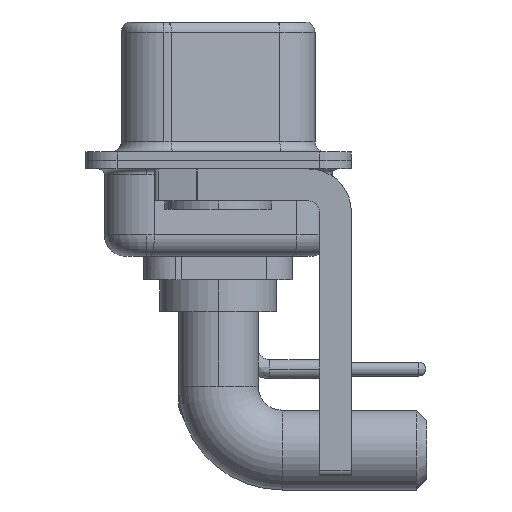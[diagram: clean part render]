
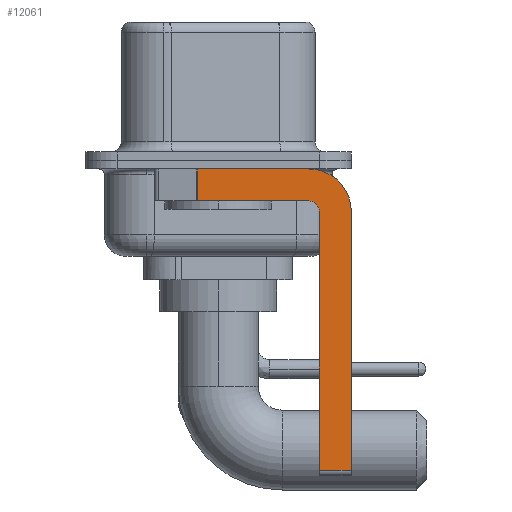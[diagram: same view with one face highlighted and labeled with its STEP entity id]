
A CAD part, left-side view. The second image highlights one B-rep face of the part: STEP entity #12061.
In plain terms, the highlighted planar face has unit normal (-1, 0, 0).
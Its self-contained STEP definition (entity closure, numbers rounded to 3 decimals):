
#58 = VERTEX_POINT ( 'NONE', #26443 ) ;
#80 = LINE ( 'NONE', #25278, #1724 ) ;
#83 = DIRECTION ( 'NONE',  ( 0., 0., -1. ) ) ;
#329 = VECTOR ( 'NONE', #21263, 1000. ) ;
#444 = CARTESIAN_POINT ( 'NONE',  ( -2.9, -4.25, -1.9 ) ) ;
#538 = CARTESIAN_POINT ( 'NONE',  ( -2.9, -4.75, -2.4 ) ) ;
#853 = DIRECTION ( 'NONE',  ( 0., 0., -1. ) ) ;
#1160 = ORIENTED_EDGE ( 'NONE', *, *, #6592, .F. ) ;
#1216 = DIRECTION ( 'NONE',  ( 0., 0., -1. ) ) ;
#1282 = CARTESIAN_POINT ( 'NONE',  ( -2.9, -6.25, -2.4 ) ) ;
#1724 = VECTOR ( 'NONE', #29143, 1000. ) ;
#2203 = EDGE_CURVE ( 'NONE', #13052, #23351, #20857, .T. ) ;
#2264 = EDGE_CURVE ( 'NONE', #17189, #18093, #7970, .T. ) ;
#3204 = CARTESIAN_POINT ( 'NONE',  ( -2.9, -4.25, -1.9 ) ) ;
#3882 = PLANE ( 'NONE',  #27304 ) ;
#5233 = VECTOR ( 'NONE', #12384, 1000. ) ;
#5284 = VERTEX_POINT ( 'NONE', #444 ) ;
#5597 = VERTEX_POINT ( 'NONE', #22332 ) ;
#5602 = CARTESIAN_POINT ( 'NONE',  ( -2.9, 0.978, -1.9 ) ) ;
#5744 = CARTESIAN_POINT ( 'NONE',  ( -2.9, -4.75, -14.8 ) ) ;
#6418 = ORIENTED_EDGE ( 'NONE', *, *, #2264, .F. ) ;
#6592 = EDGE_CURVE ( 'NONE', #5284, #23351, #21405, .T. ) ;
#7970 = LINE ( 'NONE', #5744, #10066 ) ;
#8335 = FACE_OUTER_BOUND ( 'NONE', #23864, .T. ) ;
#8390 = LINE ( 'NONE', #1282, #5233 ) ;
#8641 = EDGE_CURVE ( 'NONE', #58, #23050, #8390, .T. ) ;
#9135 = CARTESIAN_POINT ( 'NONE',  ( -2.9, -4.25, -2.4 ) ) ;
#9837 = ORIENTED_EDGE ( 'NONE', *, *, #27837, .F. ) ;
#10066 = VECTOR ( 'NONE', #14750, 1000. ) ;
#10176 = AXIS2_PLACEMENT_3D ( 'NONE', #28525, #28380, #28242 ) ;
#11211 = DIRECTION ( 'NONE',  ( 1., 0., 0. ) ) ;
#11667 = ORIENTED_EDGE ( 'NONE', *, *, #2203, .T. ) ;
#12061 = ADVANCED_FACE ( 'NONE', ( #8335 ), #3882, .F. ) ;
#12384 = DIRECTION ( 'NONE',  ( 0., 0., -1. ) ) ;
#13052 = VERTEX_POINT ( 'NONE', #17285 ) ;
#13055 = CARTESIAN_POINT ( 'NONE',  ( -2.9, -4.25, -2.4 ) ) ;
#14750 = DIRECTION ( 'NONE',  ( 0., 0., 1. ) ) ;
#15418 = LINE ( 'NONE', #21806, #25431 ) ;
#15426 = CIRCLE ( 'NONE', #18769, 2. ) ;
#17189 = VERTEX_POINT ( 'NONE', #27289 ) ;
#17285 = CARTESIAN_POINT ( 'NONE',  ( -2.9, 0.978, -0.4 ) ) ;
#17365 = DIRECTION ( 'NONE',  ( 1., 0., 0. ) ) ;
#17919 = EDGE_CURVE ( 'NONE', #13052, #5597, #15418, .T. ) ;
#18093 = VERTEX_POINT ( 'NONE', #538 ) ;
#18210 = CIRCLE ( 'NONE', #10176, 0.5 ) ;
#18769 = AXIS2_PLACEMENT_3D ( 'NONE', #9135, #11211, #83 ) ;
#19111 = CARTESIAN_POINT ( 'NONE',  ( -2.9, -6.25, -14.55 ) ) ;
#20632 = EDGE_CURVE ( 'NONE', #18093, #5284, #18210, .T. ) ;
#20857 = LINE ( 'NONE', #5602, #26624 ) ;
#21263 = DIRECTION ( 'NONE',  ( 0., 1., 0. ) ) ;
#21405 = LINE ( 'NONE', #3204, #329 ) ;
#21806 = CARTESIAN_POINT ( 'NONE',  ( -2.9, 3., -0.4 ) ) ;
#22332 = CARTESIAN_POINT ( 'NONE',  ( -2.9, -4.25, -0.4 ) ) ;
#23050 = VERTEX_POINT ( 'NONE', #19111 ) ;
#23351 = VERTEX_POINT ( 'NONE', #24565 ) ;
#23864 = EDGE_LOOP ( 'NONE', ( #26809, #11667, #1160, #28335, #6418, #25082, #28978, #9837 ) ) ;
#24304 = DIRECTION ( 'NONE',  ( 0., -1., 0. ) ) ;
#24565 = CARTESIAN_POINT ( 'NONE',  ( -2.9, 0.978, -1.9 ) ) ;
#25082 = ORIENTED_EDGE ( 'NONE', *, *, #26434, .T. ) ;
#25278 = CARTESIAN_POINT ( 'NONE',  ( -2.9, -4.25, -14.55 ) ) ;
#25431 = VECTOR ( 'NONE', #24304, 1000. ) ;
#26434 = EDGE_CURVE ( 'NONE', #17189, #23050, #80, .T. ) ;
#26443 = CARTESIAN_POINT ( 'NONE',  ( -2.9, -6.25, -2.4 ) ) ;
#26624 = VECTOR ( 'NONE', #853, 1000. ) ;
#26809 = ORIENTED_EDGE ( 'NONE', *, *, #17919, .F. ) ;
#27289 = CARTESIAN_POINT ( 'NONE',  ( -2.9, -4.75, -14.55 ) ) ;
#27304 = AXIS2_PLACEMENT_3D ( 'NONE', #13055, #17365, #1216 ) ;
#27837 = EDGE_CURVE ( 'NONE', #5597, #58, #15426, .T. ) ;
#28242 = DIRECTION ( 'NONE',  ( 0., 0., 1. ) ) ;
#28335 = ORIENTED_EDGE ( 'NONE', *, *, #20632, .F. ) ;
#28380 = DIRECTION ( 'NONE',  ( -1., 0., 0. ) ) ;
#28525 = CARTESIAN_POINT ( 'NONE',  ( -2.9, -4.25, -2.4 ) ) ;
#28978 = ORIENTED_EDGE ( 'NONE', *, *, #8641, .F. ) ;
#29143 = DIRECTION ( 'NONE',  ( 0., -1., 0. ) ) ;
